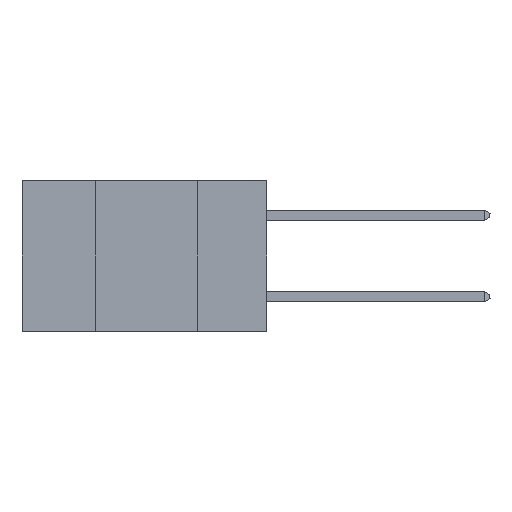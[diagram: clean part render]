
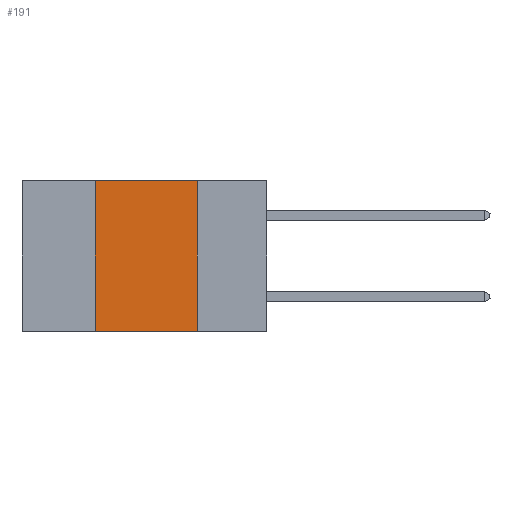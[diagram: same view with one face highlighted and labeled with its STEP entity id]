
A CAD part, left-side view. The second image highlights one B-rep face of the part: STEP entity #191.
In plain terms, the highlighted planar face has unit normal (-1, 0, 0).
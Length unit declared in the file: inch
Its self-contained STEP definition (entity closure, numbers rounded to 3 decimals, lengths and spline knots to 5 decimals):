
#191 = ADVANCED_FACE ( 'NONE', ( #29824 ), #9848, .F. ) ;
#470 = DIRECTION ( 'NONE',  ( 0., -1., 0. ) ) ;
#934 = CARTESIAN_POINT ( 'NONE',  ( 0., 0.17, -0.37 ) ) ;
#1113 = VERTEX_POINT ( 'NONE', #3747 ) ;
#1335 = VERTEX_POINT ( 'NONE', #10268 ) ;
#1435 = VECTOR ( 'NONE', #470, 39.37008 ) ;
#1835 = DIRECTION ( 'NONE',  ( 0., 0., -1. ) ) ;
#3134 = ORIENTED_EDGE ( 'NONE', *, *, #21244, .T. ) ;
#3747 = CARTESIAN_POINT ( 'NONE',  ( 0., 0.17, 0. ) ) ;
#3810 = EDGE_LOOP ( 'NONE', ( #35947, #14479, #29108, #3134 ) ) ;
#4648 = AXIS2_PLACEMENT_3D ( 'NONE', #28105, #28362, #13146 ) ;
#4802 = CARTESIAN_POINT ( 'NONE',  ( 0., 0.42, -0.37 ) ) ;
#6389 = EDGE_CURVE ( 'NONE', #1335, #1113, #36173, .T. ) ;
#7903 = CARTESIAN_POINT ( 'NONE',  ( 0., 0.17, 0. ) ) ;
#9848 = PLANE ( 'NONE',  #4648 ) ;
#10268 = CARTESIAN_POINT ( 'NONE',  ( 0., 0.42, 0. ) ) ;
#10687 = LINE ( 'NONE', #19335, #1435 ) ;
#10874 = EDGE_CURVE ( 'NONE', #14084, #1335, #39221, .T. ) ;
#13146 = DIRECTION ( 'NONE',  ( 0., 0., -1. ) ) ;
#13956 = CARTESIAN_POINT ( 'NONE',  ( 0., 0.42, 0. ) ) ;
#14084 = VERTEX_POINT ( 'NONE', #4802 ) ;
#14479 = ORIENTED_EDGE ( 'NONE', *, *, #6389, .F. ) ;
#14794 = VERTEX_POINT ( 'NONE', #934 ) ;
#15758 = VECTOR ( 'NONE', #1835, 39.37008 ) ;
#19335 = CARTESIAN_POINT ( 'NONE',  ( 0., 0.6, -0.37 ) ) ;
#21244 = EDGE_CURVE ( 'NONE', #14084, #14794, #10687, .T. ) ;
#21521 = VECTOR ( 'NONE', #32629, 39.37008 ) ;
#23191 = DIRECTION ( 'NONE',  ( 0., 0., 1. ) ) ;
#24058 = LINE ( 'NONE', #7903, #15758 ) ;
#26767 = CARTESIAN_POINT ( 'NONE',  ( 0., 0.6, 0. ) ) ;
#28105 = CARTESIAN_POINT ( 'NONE',  ( 0., 0.6, 0. ) ) ;
#28362 = DIRECTION ( 'NONE',  ( 1., 0., 0. ) ) ;
#29108 = ORIENTED_EDGE ( 'NONE', *, *, #10874, .F. ) ;
#29824 = FACE_OUTER_BOUND ( 'NONE', #3810, .T. ) ;
#32380 = VECTOR ( 'NONE', #23191, 39.37008 ) ;
#32629 = DIRECTION ( 'NONE',  ( 0., -1., 0. ) ) ;
#35525 = EDGE_CURVE ( 'NONE', #1113, #14794, #24058, .T. ) ;
#35947 = ORIENTED_EDGE ( 'NONE', *, *, #35525, .F. ) ;
#36173 = LINE ( 'NONE', #26767, #21521 ) ;
#39221 = LINE ( 'NONE', #13956, #32380 ) ;
